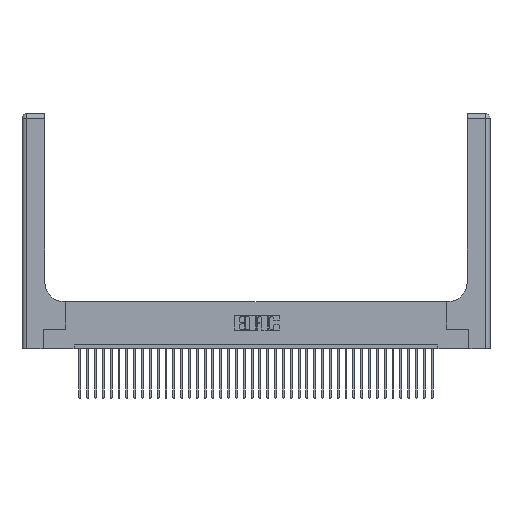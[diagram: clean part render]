
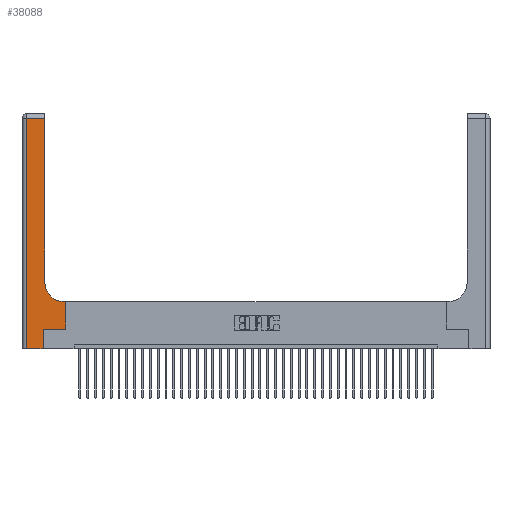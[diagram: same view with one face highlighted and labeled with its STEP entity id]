
A CAD part, top view. The second image highlights one B-rep face of the part: STEP entity #38088.
In plain terms, the highlighted planar face has unit normal (0, 0, 1).
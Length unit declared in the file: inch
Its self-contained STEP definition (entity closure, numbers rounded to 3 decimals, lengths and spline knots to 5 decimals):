
#566 = VERTEX_POINT ( 'NONE', #19212 ) ;
#940 = CARTESIAN_POINT ( 'NONE',  ( 0.06, 0., 0.37 ) ) ;
#1066 = DIRECTION ( 'NONE',  ( -1., 0., 0. ) ) ;
#1329 = ORIENTED_EDGE ( 'NONE', *, *, #13380, .T. ) ;
#1815 = EDGE_CURVE ( 'NONE', #35636, #25082, #11854, .T. ) ;
#3638 = CARTESIAN_POINT ( 'NONE',  ( 0.5585, 0.25, 0.37 ) ) ;
#4298 = DIRECTION ( 'NONE',  ( 0., -1., 0. ) ) ;
#4908 = EDGE_CURVE ( 'NONE', #25082, #34401, #31866, .T. ) ;
#5165 = ORIENTED_EDGE ( 'NONE', *, *, #19752, .T. ) ;
#5324 = AXIS2_PLACEMENT_3D ( 'NONE', #19187, #28208, #1066 ) ;
#5484 = CARTESIAN_POINT ( 'NONE',  ( 0.2915, 0.6, 0.37 ) ) ;
#6488 = VECTOR ( 'NONE', #26793, 39.37008 ) ;
#7949 = VERTEX_POINT ( 'NONE', #10269 ) ;
#7968 = ORIENTED_EDGE ( 'NONE', *, *, #20688, .T. ) ;
#8314 = LINE ( 'NONE', #13216, #21632 ) ;
#8560 = CIRCLE ( 'NONE', #35944, 0.25 ) ;
#8660 = ORIENTED_EDGE ( 'NONE', *, *, #1815, .T. ) ;
#8824 = CARTESIAN_POINT ( 'NONE',  ( 0.5585, 0.6, 0.37 ) ) ;
#9070 = DIRECTION ( 'NONE',  ( 0., 1., 0. ) ) ;
#9231 = CARTESIAN_POINT ( 'NONE',  ( 0.06, 2.94, 0.37 ) ) ;
#9828 = PLANE ( 'NONE',  #5324 ) ;
#10073 = LINE ( 'NONE', #23748, #38075 ) ;
#10269 = CARTESIAN_POINT ( 'NONE',  ( 0.2915, 0.85, 0.37 ) ) ;
#10938 = DIRECTION ( 'NONE',  ( 0., 1., 0. ) ) ;
#11060 = ORIENTED_EDGE ( 'NONE', *, *, #4908, .T. ) ;
#11090 = VERTEX_POINT ( 'NONE', #11118 ) ;
#11118 = CARTESIAN_POINT ( 'NONE',  ( 0.269, 0.25, 0.37 ) ) ;
#11854 = LINE ( 'NONE', #18821, #39303 ) ;
#11898 = VECTOR ( 'NONE', #4298, 39.37008 ) ;
#13216 = CARTESIAN_POINT ( 'NONE',  ( 0.269, 0.25, 0.37 ) ) ;
#13380 = EDGE_CURVE ( 'NONE', #11090, #17340, #8314, .T. ) ;
#14674 = LINE ( 'NONE', #5484, #6488 ) ;
#15047 = LINE ( 'NONE', #26368, #30652 ) ;
#16258 = DIRECTION ( 'NONE',  ( -1., 0., 0. ) ) ;
#17340 = VERTEX_POINT ( 'NONE', #3638 ) ;
#18819 = VECTOR ( 'NONE', #23251, 39.37008 ) ;
#18821 = CARTESIAN_POINT ( 'NONE',  ( 0., 2.94, 0.37 ) ) ;
#19187 = CARTESIAN_POINT ( 'NONE',  ( 0., 3., 0.37 ) ) ;
#19212 = CARTESIAN_POINT ( 'NONE',  ( 0.269, 0., 0.37 ) ) ;
#19213 = DIRECTION ( 'NONE',  ( 1., 0., 0. ) ) ;
#19752 = EDGE_CURVE ( 'NONE', #7949, #35636, #10073, .T. ) ;
#20688 = EDGE_CURVE ( 'NONE', #35862, #7949, #8560, .T. ) ;
#20739 = ORIENTED_EDGE ( 'NONE', *, *, #28029, .T. ) ;
#21632 = VECTOR ( 'NONE', #19213, 39.37008 ) ;
#21755 = LINE ( 'NONE', #25000, #25609 ) ;
#21839 = DIRECTION ( 'NONE',  ( 1., 0., 0. ) ) ;
#21912 = EDGE_CURVE ( 'NONE', #566, #11090, #21755, .T. ) ;
#22220 = DIRECTION ( 'NONE',  ( 0., 1., 0. ) ) ;
#22275 = EDGE_CURVE ( 'NONE', #36088, #35862, #14674, .T. ) ;
#22955 = CARTESIAN_POINT ( 'NONE',  ( 0.5415, 0.6, 0.37 ) ) ;
#23251 = DIRECTION ( 'NONE',  ( 1., 0., 0. ) ) ;
#23748 = CARTESIAN_POINT ( 'NONE',  ( 0.2915, 3., 0.37 ) ) ;
#25000 = CARTESIAN_POINT ( 'NONE',  ( 0.269, 0., 0.37 ) ) ;
#25082 = VERTEX_POINT ( 'NONE', #9231 ) ;
#25315 = CARTESIAN_POINT ( 'NONE',  ( 0.5415, 0.85, 0.37 ) ) ;
#25609 = VECTOR ( 'NONE', #22220, 39.37008 ) ;
#25895 = ORIENTED_EDGE ( 'NONE', *, *, #22275, .T. ) ;
#26368 = CARTESIAN_POINT ( 'NONE',  ( 0.5585, 0.25, 0.37 ) ) ;
#26793 = DIRECTION ( 'NONE',  ( -1., 0., 0. ) ) ;
#27777 = ORIENTED_EDGE ( 'NONE', *, *, #21912, .T. ) ;
#27853 = LINE ( 'NONE', #29357, #18819 ) ;
#27955 = DIRECTION ( 'NONE',  ( 0., 0., -1. ) ) ;
#28029 = EDGE_CURVE ( 'NONE', #34401, #566, #27853, .T. ) ;
#28208 = DIRECTION ( 'NONE',  ( 0., 0., -1. ) ) ;
#29357 = CARTESIAN_POINT ( 'NONE',  ( 0., 0., 0.37 ) ) ;
#30652 = VECTOR ( 'NONE', #10938, 39.37008 ) ;
#31866 = LINE ( 'NONE', #37579, #11898 ) ;
#34401 = VERTEX_POINT ( 'NONE', #940 ) ;
#35087 = EDGE_LOOP ( 'NONE', ( #5165, #8660, #11060, #20739, #27777, #1329, #36446, #25895, #7968 ) ) ;
#35636 = VERTEX_POINT ( 'NONE', #36656 ) ;
#35862 = VERTEX_POINT ( 'NONE', #22955 ) ;
#35944 = AXIS2_PLACEMENT_3D ( 'NONE', #25315, #27955, #21839 ) ;
#36088 = VERTEX_POINT ( 'NONE', #8824 ) ;
#36383 = EDGE_CURVE ( 'NONE', #17340, #36088, #15047, .T. ) ;
#36446 = ORIENTED_EDGE ( 'NONE', *, *, #36383, .T. ) ;
#36656 = CARTESIAN_POINT ( 'NONE',  ( 0.2915, 2.94, 0.37 ) ) ;
#36964 = FACE_OUTER_BOUND ( 'NONE', #35087, .T. ) ;
#37579 = CARTESIAN_POINT ( 'NONE',  ( 0.06, 3., 0.37 ) ) ;
#38075 = VECTOR ( 'NONE', #9070, 39.37008 ) ;
#38088 = ADVANCED_FACE ( 'NONE', ( #36964 ), #9828, .F. ) ;
#39303 = VECTOR ( 'NONE', #16258, 39.37008 ) ;
